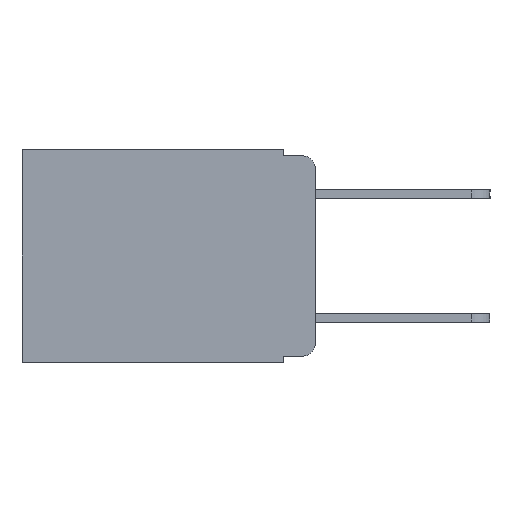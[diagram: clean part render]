
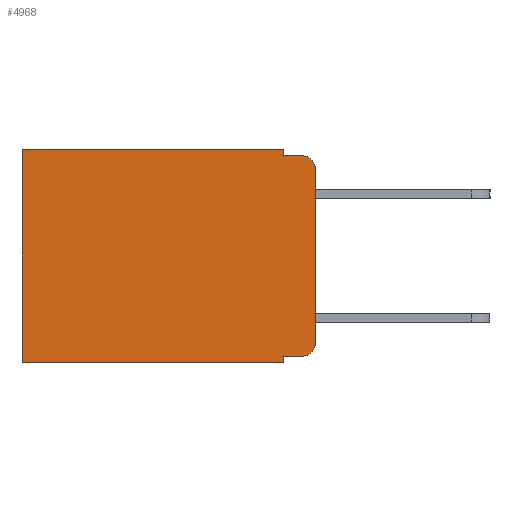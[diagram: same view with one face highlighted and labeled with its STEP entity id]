
A CAD part, left-side view. The second image highlights one B-rep face of the part: STEP entity #4968.
In plain terms, the highlighted planar face has unit normal (-1, 0, 0).
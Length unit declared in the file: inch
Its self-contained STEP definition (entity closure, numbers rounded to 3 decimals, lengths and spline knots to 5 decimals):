
#146 = VECTOR ( 'NONE', #6415, 39.37008 ) ;
#337 = CIRCLE ( 'NONE', #4255, 0.02 ) ;
#356 = VERTEX_POINT ( 'NONE', #9488 ) ;
#468 = ORIENTED_EDGE ( 'NONE', *, *, #10171, .T. ) ;
#620 = ORIENTED_EDGE ( 'NONE', *, *, #5907, .F. ) ;
#811 = ORIENTED_EDGE ( 'NONE', *, *, #10999, .F. ) ;
#1413 = VECTOR ( 'NONE', #12651, 39.37008 ) ;
#1553 = LINE ( 'NONE', #12114, #12798 ) ;
#1606 = CARTESIAN_POINT ( 'NONE',  ( 0.298, 0., -0.313 ) ) ;
#1613 = FACE_OUTER_BOUND ( 'NONE', #7598, .T. ) ;
#1950 = LINE ( 'NONE', #12169, #4095 ) ;
#2144 = ORIENTED_EDGE ( 'NONE', *, *, #3658, .T. ) ;
#2280 = VERTEX_POINT ( 'NONE', #11796 ) ;
#2377 = VECTOR ( 'NONE', #7216, 39.37008 ) ;
#2744 = LINE ( 'NONE', #6099, #2377 ) ;
#3103 = CARTESIAN_POINT ( 'NONE',  ( 0.298, 0.051, -0.343 ) ) ;
#3435 = LINE ( 'NONE', #11597, #5869 ) ;
#3654 = DIRECTION ( 'NONE',  ( 1., 0., 0. ) ) ;
#3658 = EDGE_CURVE ( 'NONE', #2280, #12645, #3435, .T. ) ;
#3745 = DIRECTION ( 'NONE',  ( 0., -1., 0. ) ) ;
#4095 = VECTOR ( 'NONE', #13133, 39.37008 ) ;
#4255 = AXIS2_PLACEMENT_3D ( 'NONE', #9941, #9953, #8185 ) ;
#4353 = EDGE_CURVE ( 'NONE', #10205, #8876, #337, .T. ) ;
#4630 = ORIENTED_EDGE ( 'NONE', *, *, #13267, .F. ) ;
#4646 = CARTESIAN_POINT ( 'NONE',  ( 0.298, 0.473, 0. ) ) ;
#4813 = VERTEX_POINT ( 'NONE', #8859 ) ;
#4968 = ADVANCED_FACE ( 'NONE', ( #1613 ), #7589, .F. ) ;
#5086 = VECTOR ( 'NONE', #13248, 39.37008 ) ;
#5166 = EDGE_CURVE ( 'NONE', #4813, #10205, #13649, .T. ) ;
#5610 = CARTESIAN_POINT ( 'NONE',  ( 0.298, 0.02, -0.03 ) ) ;
#5714 = DIRECTION ( 'NONE',  ( 0., -1., 0. ) ) ;
#5869 = VECTOR ( 'NONE', #7678, 39.37008 ) ;
#5907 = EDGE_CURVE ( 'NONE', #4813, #7681, #9630, .T. ) ;
#6018 = AXIS2_PLACEMENT_3D ( 'NONE', #13502, #3654, #10681 ) ;
#6099 = CARTESIAN_POINT ( 'NONE',  ( 0.298, 0., -0.343 ) ) ;
#6415 = DIRECTION ( 'NONE',  ( 0., 0., -1. ) ) ;
#6474 = CARTESIAN_POINT ( 'NONE',  ( 0.298, 0.473, -0.343 ) ) ;
#6528 = LINE ( 'NONE', #12791, #146 ) ;
#6708 = DIRECTION ( 'NONE',  ( 0., 0., -1. ) ) ;
#6824 = CIRCLE ( 'NONE', #13787, 0.02 ) ;
#7143 = ORIENTED_EDGE ( 'NONE', *, *, #8867, .F. ) ;
#7216 = DIRECTION ( 'NONE',  ( 0., 1., 0. ) ) ;
#7259 = CARTESIAN_POINT ( 'NONE',  ( 0.298, 0.02, -0.01 ) ) ;
#7589 = PLANE ( 'NONE',  #6018 ) ;
#7598 = EDGE_LOOP ( 'NONE', ( #7143, #468, #9546, #811, #2144, #11649, #4630, #620, #13162, #11682 ) ) ;
#7678 = DIRECTION ( 'NONE',  ( 0., 1., 0. ) ) ;
#7681 = VERTEX_POINT ( 'NONE', #3103 ) ;
#7689 = LINE ( 'NONE', #4646, #5086 ) ;
#8010 = CARTESIAN_POINT ( 'NONE',  ( 0.298, 0.051, -0.333 ) ) ;
#8081 = VECTOR ( 'NONE', #3745, 39.37008 ) ;
#8185 = DIRECTION ( 'NONE',  ( 0., 0., -1. ) ) ;
#8252 = VERTEX_POINT ( 'NONE', #6474 ) ;
#8287 = CARTESIAN_POINT ( 'NONE',  ( 0.298, 0.473, 0. ) ) ;
#8859 = CARTESIAN_POINT ( 'NONE',  ( 0.298, 0.051, -0.333 ) ) ;
#8867 = EDGE_CURVE ( 'NONE', #9537, #8876, #6528, .T. ) ;
#8876 = VERTEX_POINT ( 'NONE', #1606 ) ;
#8899 = CARTESIAN_POINT ( 'NONE',  ( 0.298, 0., -0.03 ) ) ;
#9488 = CARTESIAN_POINT ( 'NONE',  ( 0.298, 0.051, -0.01 ) ) ;
#9537 = VERTEX_POINT ( 'NONE', #8899 ) ;
#9546 = ORIENTED_EDGE ( 'NONE', *, *, #13738, .F. ) ;
#9630 = LINE ( 'NONE', #11181, #1413 ) ;
#9941 = CARTESIAN_POINT ( 'NONE',  ( 0.298, 0.02, -0.313 ) ) ;
#9953 = DIRECTION ( 'NONE',  ( -1., 0., 0. ) ) ;
#10171 = EDGE_CURVE ( 'NONE', #9537, #13301, #6824, .T. ) ;
#10205 = VERTEX_POINT ( 'NONE', #13110 ) ;
#10308 = EDGE_CURVE ( 'NONE', #12645, #8252, #7689, .T. ) ;
#10681 = DIRECTION ( 'NONE',  ( 0., 0., -1. ) ) ;
#10999 = EDGE_CURVE ( 'NONE', #2280, #356, #1950, .T. ) ;
#11181 = CARTESIAN_POINT ( 'NONE',  ( 0.298, 0.051, 0. ) ) ;
#11597 = CARTESIAN_POINT ( 'NONE',  ( 0.298, 0., 0. ) ) ;
#11649 = ORIENTED_EDGE ( 'NONE', *, *, #10308, .T. ) ;
#11682 = ORIENTED_EDGE ( 'NONE', *, *, #4353, .T. ) ;
#11796 = CARTESIAN_POINT ( 'NONE',  ( 0.298, 0.051, 0. ) ) ;
#12114 = CARTESIAN_POINT ( 'NONE',  ( 0.298, 0.051, -0.01 ) ) ;
#12169 = CARTESIAN_POINT ( 'NONE',  ( 0.298, 0.051, 0. ) ) ;
#12645 = VERTEX_POINT ( 'NONE', #8287 ) ;
#12651 = DIRECTION ( 'NONE',  ( 0., 0., -1. ) ) ;
#12791 = CARTESIAN_POINT ( 'NONE',  ( 0.298, 0., 0. ) ) ;
#12798 = VECTOR ( 'NONE', #5714, 39.37008 ) ;
#13067 = DIRECTION ( 'NONE',  ( -1., 0., 0. ) ) ;
#13110 = CARTESIAN_POINT ( 'NONE',  ( 0.298, 0.02, -0.333 ) ) ;
#13133 = DIRECTION ( 'NONE',  ( 0., 0., -1. ) ) ;
#13162 = ORIENTED_EDGE ( 'NONE', *, *, #5166, .T. ) ;
#13248 = DIRECTION ( 'NONE',  ( 0., 0., -1. ) ) ;
#13267 = EDGE_CURVE ( 'NONE', #7681, #8252, #2744, .T. ) ;
#13301 = VERTEX_POINT ( 'NONE', #7259 ) ;
#13502 = CARTESIAN_POINT ( 'NONE',  ( 0.298, 0., 0. ) ) ;
#13649 = LINE ( 'NONE', #8010, #8081 ) ;
#13738 = EDGE_CURVE ( 'NONE', #356, #13301, #1553, .T. ) ;
#13787 = AXIS2_PLACEMENT_3D ( 'NONE', #5610, #13067, #6708 ) ;
